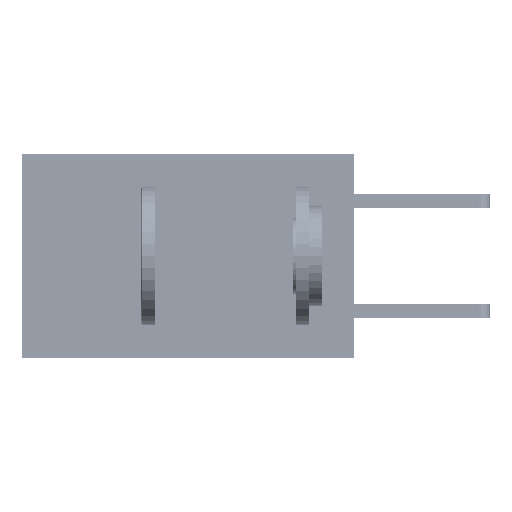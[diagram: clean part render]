
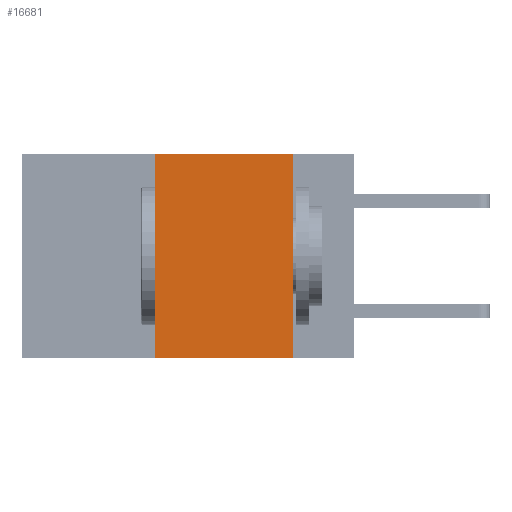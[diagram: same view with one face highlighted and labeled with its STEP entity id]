
A CAD part, left-side view. The second image highlights one B-rep face of the part: STEP entity #16681.
In plain terms, the highlighted planar face has unit normal (-1, 0, 0).
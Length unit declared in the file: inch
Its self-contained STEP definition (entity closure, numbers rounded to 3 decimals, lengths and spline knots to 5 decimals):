
#946 = DIRECTION ( 'NONE',  ( 0., 0., -1. ) ) ;
#1434 = DIRECTION ( 'NONE',  ( 0., -1., 0. ) ) ;
#1706 = EDGE_CURVE ( 'NONE', #26388, #33159, #7431, .T. ) ;
#3312 = LINE ( 'NONE', #17242, #4331 ) ;
#4331 = VECTOR ( 'NONE', #946, 39.37008 ) ;
#5215 = CARTESIAN_POINT ( 'NONE',  ( 0., 0.36, 0. ) ) ;
#5703 = CARTESIAN_POINT ( 'NONE',  ( 0., 0.36, 0. ) ) ;
#5987 = DIRECTION ( 'NONE',  ( 0., 0., 1. ) ) ;
#7327 = CARTESIAN_POINT ( 'NONE',  ( 0., 0.6, -0.37 ) ) ;
#7431 = LINE ( 'NONE', #7327, #14740 ) ;
#9579 = PLANE ( 'NONE',  #28453 ) ;
#12017 = ORIENTED_EDGE ( 'NONE', *, *, #19990, .F. ) ;
#12941 = CARTESIAN_POINT ( 'NONE',  ( 0., 0.6, 0. ) ) ;
#13153 = CARTESIAN_POINT ( 'NONE',  ( 0., 0.11, -0.37 ) ) ;
#13514 = FACE_OUTER_BOUND ( 'NONE', #23277, .T. ) ;
#14319 = CARTESIAN_POINT ( 'NONE',  ( 0., 0.36, -0.37 ) ) ;
#14740 = VECTOR ( 'NONE', #1434, 39.37008 ) ;
#15820 = CARTESIAN_POINT ( 'NONE',  ( 0., 0.11, 0. ) ) ;
#16681 = ADVANCED_FACE ( 'NONE', ( #13514 ), #9579, .F. ) ;
#17242 = CARTESIAN_POINT ( 'NONE',  ( 0., 0.11, 0. ) ) ;
#18957 = VECTOR ( 'NONE', #21596, 39.37008 ) ;
#19233 = ORIENTED_EDGE ( 'NONE', *, *, #32411, .F. ) ;
#19553 = EDGE_CURVE ( 'NONE', #30731, #33159, #3312, .T. ) ;
#19990 = EDGE_CURVE ( 'NONE', #33849, #30731, #26273, .T. ) ;
#21596 = DIRECTION ( 'NONE',  ( 0., -1., 0. ) ) ;
#22388 = DIRECTION ( 'NONE',  ( 0., 0., -1. ) ) ;
#23277 = EDGE_LOOP ( 'NONE', ( #42211, #12017, #19233, #37645 ) ) ;
#25788 = DIRECTION ( 'NONE',  ( 1., 0., 0. ) ) ;
#26273 = LINE ( 'NONE', #35441, #18957 ) ;
#26388 = VERTEX_POINT ( 'NONE', #14319 ) ;
#28453 = AXIS2_PLACEMENT_3D ( 'NONE', #12941, #25788, #22388 ) ;
#30731 = VERTEX_POINT ( 'NONE', #15820 ) ;
#32411 = EDGE_CURVE ( 'NONE', #26388, #33849, #40821, .T. ) ;
#33159 = VERTEX_POINT ( 'NONE', #13153 ) ;
#33849 = VERTEX_POINT ( 'NONE', #5215 ) ;
#35441 = CARTESIAN_POINT ( 'NONE',  ( 0., 0.6, 0. ) ) ;
#37645 = ORIENTED_EDGE ( 'NONE', *, *, #1706, .T. ) ;
#40821 = LINE ( 'NONE', #5703, #41878 ) ;
#41878 = VECTOR ( 'NONE', #5987, 39.37008 ) ;
#42211 = ORIENTED_EDGE ( 'NONE', *, *, #19553, .F. ) ;
